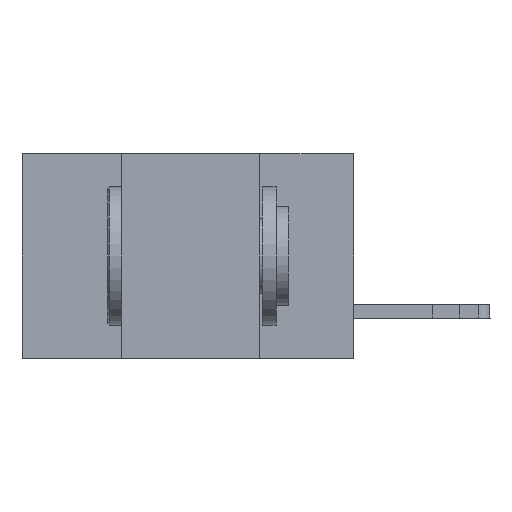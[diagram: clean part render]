
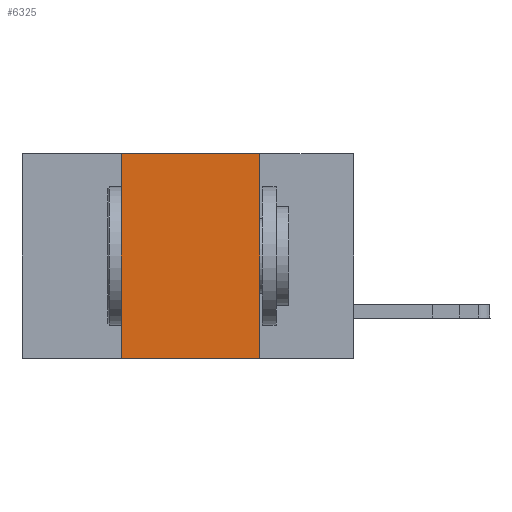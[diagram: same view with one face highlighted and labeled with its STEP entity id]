
A CAD part, left-side view. The second image highlights one B-rep face of the part: STEP entity #6325.
In plain terms, the highlighted planar face has unit normal (-1, 0, 0).
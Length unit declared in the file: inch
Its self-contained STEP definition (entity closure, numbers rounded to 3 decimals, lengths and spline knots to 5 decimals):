
#215 = ORIENTED_EDGE ( 'NONE', *, *, #24299, .F. ) ;
#1252 = EDGE_CURVE ( 'NONE', #17268, #37219, #29125, .T. ) ;
#1452 = CARTESIAN_POINT ( 'NONE',  ( 0., 0.6, 0. ) ) ;
#2092 = DIRECTION ( 'NONE',  ( 0., 0., 1. ) ) ;
#4733 = VECTOR ( 'NONE', #20222, 39.37008 ) ;
#6325 = ADVANCED_FACE ( 'NONE', ( #22477 ), #33998, .F. ) ;
#6379 = VECTOR ( 'NONE', #2092, 39.37008 ) ;
#8304 = DIRECTION ( 'NONE',  ( 0., 0., -1. ) ) ;
#11615 = ORIENTED_EDGE ( 'NONE', *, *, #1252, .T. ) ;
#11841 = CARTESIAN_POINT ( 'NONE',  ( 0., 0.17, -0.37 ) ) ;
#12773 = LINE ( 'NONE', #1452, #31467 ) ;
#16578 = CARTESIAN_POINT ( 'NONE',  ( 0., 0.42, 0. ) ) ;
#16955 = LINE ( 'NONE', #19207, #25980 ) ;
#17268 = VERTEX_POINT ( 'NONE', #36956 ) ;
#17321 = EDGE_CURVE ( 'NONE', #28176, #37219, #16955, .T. ) ;
#18584 = DIRECTION ( 'NONE',  ( 0., -1., 0. ) ) ;
#18909 = CARTESIAN_POINT ( 'NONE',  ( 0., 0.6, 0. ) ) ;
#19207 = CARTESIAN_POINT ( 'NONE',  ( 0., 0.17, 0. ) ) ;
#20222 = DIRECTION ( 'NONE',  ( 0., -1., 0. ) ) ;
#20612 = CARTESIAN_POINT ( 'NONE',  ( 0., 0.6, -0.37 ) ) ;
#21173 = EDGE_LOOP ( 'NONE', ( #35471, #215, #21298, #11615 ) ) ;
#21298 = ORIENTED_EDGE ( 'NONE', *, *, #29944, .F. ) ;
#22102 = DIRECTION ( 'NONE',  ( 1., 0., 0. ) ) ;
#22477 = FACE_OUTER_BOUND ( 'NONE', #21173, .T. ) ;
#24299 = EDGE_CURVE ( 'NONE', #29850, #28176, #12773, .T. ) ;
#25980 = VECTOR ( 'NONE', #8304, 39.37008 ) ;
#27178 = CARTESIAN_POINT ( 'NONE',  ( 0., 0.42, 0. ) ) ;
#28034 = AXIS2_PLACEMENT_3D ( 'NONE', #18909, #22102, #30822 ) ;
#28176 = VERTEX_POINT ( 'NONE', #33917 ) ;
#29125 = LINE ( 'NONE', #20612, #4733 ) ;
#29850 = VERTEX_POINT ( 'NONE', #27178 ) ;
#29944 = EDGE_CURVE ( 'NONE', #17268, #29850, #30943, .T. ) ;
#30822 = DIRECTION ( 'NONE',  ( 0., 0., -1. ) ) ;
#30943 = LINE ( 'NONE', #16578, #6379 ) ;
#31467 = VECTOR ( 'NONE', #18584, 39.37008 ) ;
#33917 = CARTESIAN_POINT ( 'NONE',  ( 0., 0.17, 0. ) ) ;
#33998 = PLANE ( 'NONE',  #28034 ) ;
#35471 = ORIENTED_EDGE ( 'NONE', *, *, #17321, .F. ) ;
#36956 = CARTESIAN_POINT ( 'NONE',  ( 0., 0.42, -0.37 ) ) ;
#37219 = VERTEX_POINT ( 'NONE', #11841 ) ;
